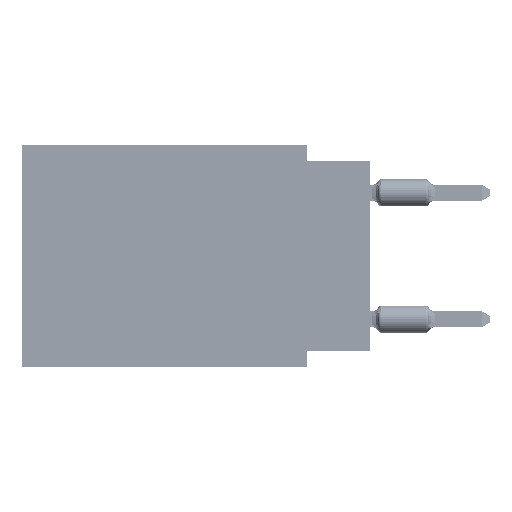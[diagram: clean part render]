
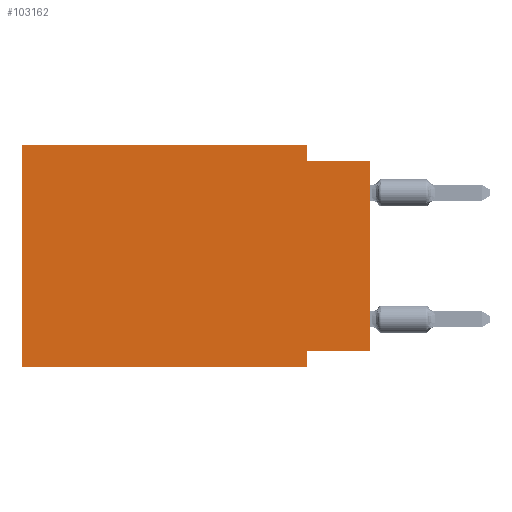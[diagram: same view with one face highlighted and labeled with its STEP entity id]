
A CAD part, left-side view. The second image highlights one B-rep face of the part: STEP entity #103162.
In plain terms, the highlighted planar face has unit normal (-1, 0, 0).
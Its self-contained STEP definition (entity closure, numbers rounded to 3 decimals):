
#4310 = CARTESIAN_POINT ( 'NONE',  ( 0., 13.97, 0. ) ) ;
#5341 = LINE ( 'NONE', #112584, #12836 ) ;
#5999 = ORIENTED_EDGE ( 'NONE', *, *, #16473, .F. ) ;
#7827 = DIRECTION ( 'NONE',  ( 0., 1., 0. ) ) ;
#8459 = CARTESIAN_POINT ( 'NONE',  ( 0., 13.97, 0. ) ) ;
#9394 = VECTOR ( 'NONE', #89139, 1000. ) ;
#10415 = LINE ( 'NONE', #10996, #48912 ) ;
#10996 = CARTESIAN_POINT ( 'NONE',  ( 0., 0., -0.635 ) ) ;
#12093 = VERTEX_POINT ( 'NONE', #8459 ) ;
#12679 = VECTOR ( 'NONE', #40796, 1000. ) ;
#12836 = VECTOR ( 'NONE', #32312, 1000. ) ;
#16473 = EDGE_CURVE ( 'NONE', #19157, #38881, #81063, .T. ) ;
#18676 = ORIENTED_EDGE ( 'NONE', *, *, #47711, .F. ) ;
#19157 = VERTEX_POINT ( 'NONE', #91767 ) ;
#19362 = CARTESIAN_POINT ( 'NONE',  ( 0., 2.54, -8.255 ) ) ;
#25169 = VECTOR ( 'NONE', #7827, 1000. ) ;
#25524 = ORIENTED_EDGE ( 'NONE', *, *, #56238, .F. ) ;
#27463 = VERTEX_POINT ( 'NONE', #83780 ) ;
#29059 = VECTOR ( 'NONE', #96511, 1000. ) ;
#30052 = VERTEX_POINT ( 'NONE', #104705 ) ;
#30571 = CARTESIAN_POINT ( 'NONE',  ( 0., 2.54, -0.635 ) ) ;
#32312 = DIRECTION ( 'NONE',  ( 0., 0., 1. ) ) ;
#33788 = EDGE_CURVE ( 'NONE', #61533, #39734, #10415, .T. ) ;
#34485 = CARTESIAN_POINT ( 'NONE',  ( 0., 2.54, -8.89 ) ) ;
#34669 = ORIENTED_EDGE ( 'NONE', *, *, #94387, .T. ) ;
#34781 = VERTEX_POINT ( 'NONE', #93317 ) ;
#35737 = ORIENTED_EDGE ( 'NONE', *, *, #45852, .F. ) ;
#37441 = VECTOR ( 'NONE', #62769, 1000. ) ;
#37562 = CARTESIAN_POINT ( 'NONE',  ( 0., 13.97, -8.89 ) ) ;
#38881 = VERTEX_POINT ( 'NONE', #19362 ) ;
#39734 = VERTEX_POINT ( 'NONE', #54270 ) ;
#40005 = EDGE_LOOP ( 'NONE', ( #66842, #70142, #101031, #25524, #35737, #34669, #18676, #5999 ) ) ;
#40227 = LINE ( 'NONE', #104072, #12679 ) ;
#40796 = DIRECTION ( 'NONE',  ( 0., 0., -1. ) ) ;
#45852 = EDGE_CURVE ( 'NONE', #30052, #12093, #5341, .T. ) ;
#46333 = LINE ( 'NONE', #71560, #37441 ) ;
#47711 = EDGE_CURVE ( 'NONE', #38881, #27463, #114766, .T. ) ;
#48912 = VECTOR ( 'NONE', #81909, 1000. ) ;
#52388 = CARTESIAN_POINT ( 'NONE',  ( 0., 0., -8.255 ) ) ;
#53153 = CARTESIAN_POINT ( 'NONE',  ( 0., 13.97, 0. ) ) ;
#54270 = CARTESIAN_POINT ( 'NONE',  ( 0., 0., -0.635 ) ) ;
#56238 = EDGE_CURVE ( 'NONE', #12093, #34781, #115242, .T. ) ;
#57640 = DIRECTION ( 'NONE',  ( 0., 0., -1. ) ) ;
#61533 = VERTEX_POINT ( 'NONE', #30571 ) ;
#62769 = DIRECTION ( 'NONE',  ( 0., 0., 1. ) ) ;
#66842 = ORIENTED_EDGE ( 'NONE', *, *, #94395, .T. ) ;
#67012 = DIRECTION ( 'NONE',  ( 1., 0., 0. ) ) ;
#70142 = ORIENTED_EDGE ( 'NONE', *, *, #33788, .F. ) ;
#70219 = DIRECTION ( 'NONE',  ( 0., 0., -1. ) ) ;
#71560 = CARTESIAN_POINT ( 'NONE',  ( 0., 0., 0. ) ) ;
#73789 = AXIS2_PLACEMENT_3D ( 'NONE', #4310, #67012, #57640 ) ;
#81063 = LINE ( 'NONE', #52388, #25169 ) ;
#81909 = DIRECTION ( 'NONE',  ( 0., -1., 0. ) ) ;
#82080 = LINE ( 'NONE', #37562, #9394 ) ;
#83435 = PLANE ( 'NONE',  #73789 ) ;
#83780 = CARTESIAN_POINT ( 'NONE',  ( 0., 2.54, -8.89 ) ) ;
#89139 = DIRECTION ( 'NONE',  ( 0., -1., 0. ) ) ;
#91767 = CARTESIAN_POINT ( 'NONE',  ( 0., 0., -8.255 ) ) ;
#93317 = CARTESIAN_POINT ( 'NONE',  ( 0., 2.54, 0. ) ) ;
#94387 = EDGE_CURVE ( 'NONE', #30052, #27463, #82080, .T. ) ;
#94395 = EDGE_CURVE ( 'NONE', #19157, #39734, #46333, .T. ) ;
#96511 = DIRECTION ( 'NONE',  ( 0., -1., 0. ) ) ;
#100830 = VECTOR ( 'NONE', #70219, 1000. ) ;
#101031 = ORIENTED_EDGE ( 'NONE', *, *, #111543, .F. ) ;
#103162 = ADVANCED_FACE ( 'NONE', ( #110398 ), #83435, .F. ) ;
#104072 = CARTESIAN_POINT ( 'NONE',  ( 0., 2.54, 0. ) ) ;
#104705 = CARTESIAN_POINT ( 'NONE',  ( 0., 13.97, -8.89 ) ) ;
#110398 = FACE_OUTER_BOUND ( 'NONE', #40005, .T. ) ;
#111543 = EDGE_CURVE ( 'NONE', #34781, #61533, #40227, .T. ) ;
#112584 = CARTESIAN_POINT ( 'NONE',  ( 0., 13.97, 0. ) ) ;
#114766 = LINE ( 'NONE', #34485, #100830 ) ;
#115242 = LINE ( 'NONE', #53153, #29059 ) ;
